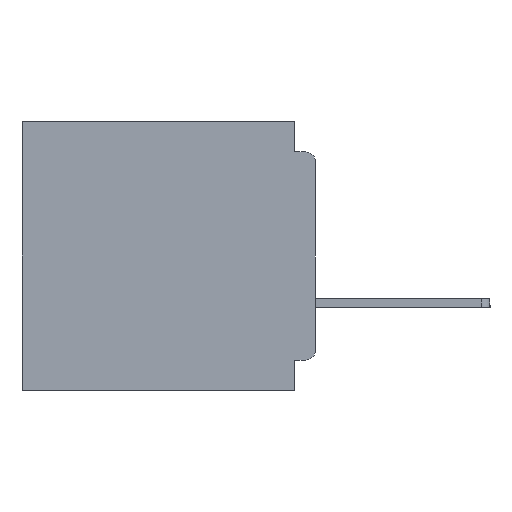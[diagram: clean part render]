
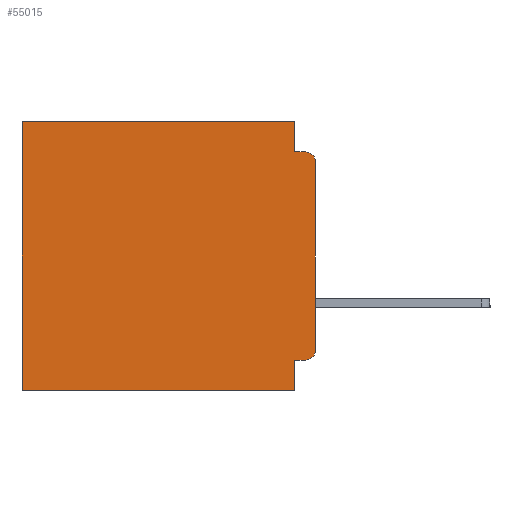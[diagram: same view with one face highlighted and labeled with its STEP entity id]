
A CAD part, left-side view. The second image highlights one B-rep face of the part: STEP entity #55015.
In plain terms, the highlighted planar face has unit normal (-1, 0, 0).
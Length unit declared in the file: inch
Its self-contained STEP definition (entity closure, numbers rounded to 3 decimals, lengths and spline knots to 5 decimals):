
#254 = CARTESIAN_POINT ( 'NONE',  ( 0.3, 0.031, -0.4 ) ) ;
#877 = LINE ( 'NONE', #29518, #11253 ) ;
#932 = CARTESIAN_POINT ( 'NONE',  ( 0.3, 0.031, 0. ) ) ;
#1856 = VECTOR ( 'NONE', #4360, 39.37008 ) ;
#2747 = VERTEX_POINT ( 'NONE', #30791 ) ;
#2909 = ORIENTED_EDGE ( 'NONE', *, *, #56344, .F. ) ;
#3245 = LINE ( 'NONE', #56461, #1856 ) ;
#3587 = EDGE_CURVE ( 'NONE', #41468, #47038, #45306, .T. ) ;
#4360 = DIRECTION ( 'NONE',  ( 0., 1., 0. ) ) ;
#5250 = ORIENTED_EDGE ( 'NONE', *, *, #32193, .F. ) ;
#5444 = EDGE_CURVE ( 'NONE', #33131, #8971, #11428, .T. ) ;
#5573 = CARTESIAN_POINT ( 'NONE',  ( 0.3, 0.015, -0.06 ) ) ;
#6629 = CARTESIAN_POINT ( 'NONE',  ( 0.3, 0.031, -0.4 ) ) ;
#7183 = CARTESIAN_POINT ( 'NONE',  ( 0.3, 0.015, -0.34 ) ) ;
#8716 = CARTESIAN_POINT ( 'NONE',  ( 0.3, 0.437, 0. ) ) ;
#8971 = VERTEX_POINT ( 'NONE', #9649 ) ;
#9649 = CARTESIAN_POINT ( 'NONE',  ( 0.3, 0., -0.34 ) ) ;
#10011 = DIRECTION ( 'NONE',  ( 0., 0., -1. ) ) ;
#10645 = VECTOR ( 'NONE', #40823, 39.37008 ) ;
#11044 = DIRECTION ( 'NONE',  ( 0., 0., -1. ) ) ;
#11253 = VECTOR ( 'NONE', #51027, 39.37008 ) ;
#11428 = LINE ( 'NONE', #47177, #44740 ) ;
#11572 = VERTEX_POINT ( 'NONE', #932 ) ;
#11600 = DIRECTION ( 'NONE',  ( 0., 0., -1. ) ) ;
#11985 = ORIENTED_EDGE ( 'NONE', *, *, #35838, .T. ) ;
#12005 = LINE ( 'NONE', #6629, #20934 ) ;
#12465 = FACE_OUTER_BOUND ( 'NONE', #28618, .T. ) ;
#12672 = VERTEX_POINT ( 'NONE', #35460 ) ;
#12719 = ORIENTED_EDGE ( 'NONE', *, *, #42896, .F. ) ;
#13365 = ORIENTED_EDGE ( 'NONE', *, *, #53512, .T. ) ;
#15557 = CARTESIAN_POINT ( 'NONE',  ( 0.3, 0.437, -0.4 ) ) ;
#16555 = DIRECTION ( 'NONE',  ( 0., 0., -1. ) ) ;
#16876 = ORIENTED_EDGE ( 'NONE', *, *, #5444, .F. ) ;
#18795 = AXIS2_PLACEMENT_3D ( 'NONE', #7183, #37627, #11600 ) ;
#19700 = EDGE_CURVE ( 'NONE', #32566, #38348, #12005, .T. ) ;
#20577 = VECTOR ( 'NONE', #26235, 39.37008 ) ;
#20934 = VECTOR ( 'NONE', #11044, 39.37008 ) ;
#21691 = CIRCLE ( 'NONE', #18795, 0.015 ) ;
#21890 = CARTESIAN_POINT ( 'NONE',  ( 0.3, 0.031, 0. ) ) ;
#24363 = VERTEX_POINT ( 'NONE', #8716 ) ;
#24984 = CIRCLE ( 'NONE', #50763, 0.015 ) ;
#25728 = DIRECTION ( 'NONE',  ( 1., 0., 0. ) ) ;
#26235 = DIRECTION ( 'NONE',  ( 0., 0., -1. ) ) ;
#28618 = EDGE_LOOP ( 'NONE', ( #16876, #13365, #44265, #12719, #11985, #49478, #2909, #49690, #5250, #55873 ) ) ;
#29518 = CARTESIAN_POINT ( 'NONE',  ( 0.3, 0., 0. ) ) ;
#30791 = CARTESIAN_POINT ( 'NONE',  ( 0.3, 0.437, -0.4 ) ) ;
#32026 = CARTESIAN_POINT ( 'NONE',  ( 0.3, 0., -0.045 ) ) ;
#32193 = EDGE_CURVE ( 'NONE', #12672, #32566, #3245, .T. ) ;
#32566 = VERTEX_POINT ( 'NONE', #55479 ) ;
#33131 = VERTEX_POINT ( 'NONE', #45241 ) ;
#33275 = EDGE_CURVE ( 'NONE', #12672, #8971, #21691, .T. ) ;
#34342 = EDGE_CURVE ( 'NONE', #24363, #2747, #54035, .T. ) ;
#35460 = CARTESIAN_POINT ( 'NONE',  ( 0.3, 0.015, -0.355 ) ) ;
#35838 = EDGE_CURVE ( 'NONE', #11572, #24363, #877, .T. ) ;
#36106 = DIRECTION ( 'NONE',  ( -1., 0., 0. ) ) ;
#36390 = AXIS2_PLACEMENT_3D ( 'NONE', #46319, #25728, #56000 ) ;
#37163 = CARTESIAN_POINT ( 'NONE',  ( 0.3, 0.015, -0.045 ) ) ;
#37627 = DIRECTION ( 'NONE',  ( -1., 0., 0. ) ) ;
#38348 = VERTEX_POINT ( 'NONE', #254 ) ;
#40823 = DIRECTION ( 'NONE',  ( 0., -1., 0. ) ) ;
#41468 = VERTEX_POINT ( 'NONE', #41469 ) ;
#41469 = CARTESIAN_POINT ( 'NONE',  ( 0.3, 0.031, -0.045 ) ) ;
#42160 = PLANE ( 'NONE',  #36390 ) ;
#42518 = VECTOR ( 'NONE', #54589, 39.37008 ) ;
#42896 = EDGE_CURVE ( 'NONE', #11572, #41468, #43599, .T. ) ;
#43599 = LINE ( 'NONE', #21890, #20577 ) ;
#44265 = ORIENTED_EDGE ( 'NONE', *, *, #3587, .F. ) ;
#44740 = VECTOR ( 'NONE', #16555, 39.37008 ) ;
#45241 = CARTESIAN_POINT ( 'NONE',  ( 0.3, 0., -0.06 ) ) ;
#45306 = LINE ( 'NONE', #32026, #10645 ) ;
#46319 = CARTESIAN_POINT ( 'NONE',  ( 0.3, 0., -0.4 ) ) ;
#46932 = LINE ( 'NONE', #51871, #55766 ) ;
#47038 = VERTEX_POINT ( 'NONE', #37163 ) ;
#47177 = CARTESIAN_POINT ( 'NONE',  ( 0.3, 0., -0.4 ) ) ;
#49478 = ORIENTED_EDGE ( 'NONE', *, *, #34342, .T. ) ;
#49690 = ORIENTED_EDGE ( 'NONE', *, *, #19700, .F. ) ;
#50763 = AXIS2_PLACEMENT_3D ( 'NONE', #5573, #36106, #10011 ) ;
#51027 = DIRECTION ( 'NONE',  ( 0., 1., 0. ) ) ;
#51871 = CARTESIAN_POINT ( 'NONE',  ( 0.3, 0., -0.4 ) ) ;
#53512 = EDGE_CURVE ( 'NONE', #33131, #47038, #24984, .T. ) ;
#54035 = LINE ( 'NONE', #15557, #42518 ) ;
#54589 = DIRECTION ( 'NONE',  ( 0., 0., -1. ) ) ;
#55015 = ADVANCED_FACE ( 'NONE', ( #12465 ), #42160, .F. ) ;
#55479 = CARTESIAN_POINT ( 'NONE',  ( 0.3, 0.031, -0.355 ) ) ;
#55766 = VECTOR ( 'NONE', #56228, 39.37008 ) ;
#55873 = ORIENTED_EDGE ( 'NONE', *, *, #33275, .T. ) ;
#56000 = DIRECTION ( 'NONE',  ( 0., 0., -1. ) ) ;
#56228 = DIRECTION ( 'NONE',  ( 0., 1., 0. ) ) ;
#56344 = EDGE_CURVE ( 'NONE', #38348, #2747, #46932, .T. ) ;
#56461 = CARTESIAN_POINT ( 'NONE',  ( 0.3, 0., -0.355 ) ) ;
